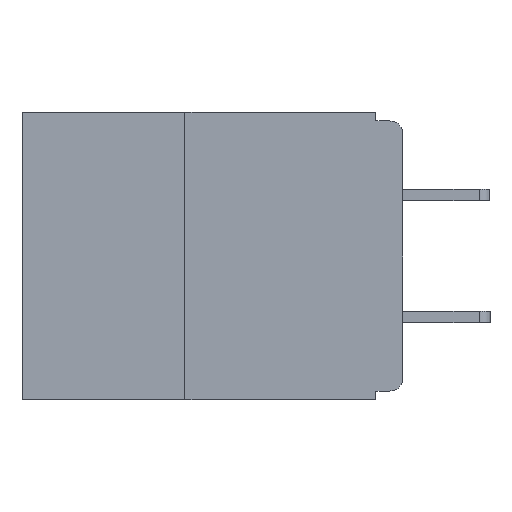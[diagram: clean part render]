
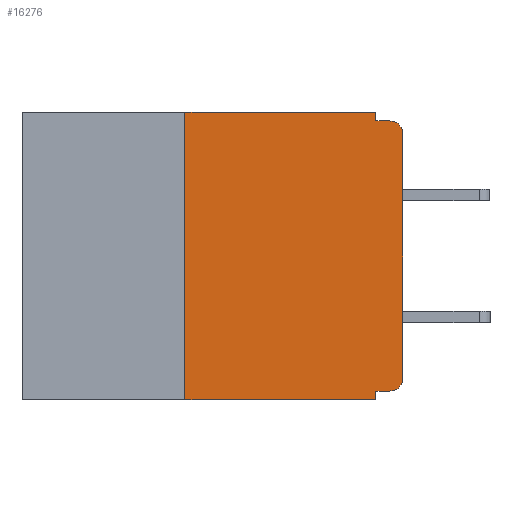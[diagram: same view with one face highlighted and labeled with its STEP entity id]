
A CAD part, left-side view. The second image highlights one B-rep face of the part: STEP entity #16276.
In plain terms, the highlighted planar face has unit normal (-1, 0, 0).
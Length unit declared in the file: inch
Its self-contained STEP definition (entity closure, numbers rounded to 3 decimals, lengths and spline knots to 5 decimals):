
#158 = CARTESIAN_POINT ( 'NONE',  ( 0., 0., -0.32 ) ) ;
#183 = VERTEX_POINT ( 'NONE', #25797 ) ;
#753 = VECTOR ( 'NONE', #14647, 39.37008 ) ;
#823 = DIRECTION ( 'NONE',  ( 0., 0., 1. ) ) ;
#882 = CARTESIAN_POINT ( 'NONE',  ( 0., 0.25, -0.33 ) ) ;
#930 = DIRECTION ( 'NONE',  ( 0., 0., -1. ) ) ;
#1083 = AXIS2_PLACEMENT_3D ( 'NONE', #5230, #19446, #7281 ) ;
#1275 = EDGE_CURVE ( 'NONE', #183, #2156, #4317, .T. ) ;
#1874 = CARTESIAN_POINT ( 'NONE',  ( 0., 0.031, -0.01 ) ) ;
#2099 = ORIENTED_EDGE ( 'NONE', *, *, #3754, .F. ) ;
#2156 = VERTEX_POINT ( 'NONE', #15948 ) ;
#2286 = DIRECTION ( 'NONE',  ( 0., 1., 0. ) ) ;
#2629 = CARTESIAN_POINT ( 'NONE',  ( 0., 0.031, -0.33 ) ) ;
#2714 = CARTESIAN_POINT ( 'NONE',  ( 0., 0.25, 0. ) ) ;
#3185 = LINE ( 'NONE', #158, #13407 ) ;
#3301 = CARTESIAN_POINT ( 'NONE',  ( 0., 0.031, 0. ) ) ;
#3754 = EDGE_CURVE ( 'NONE', #14753, #25849, #5855, .T. ) ;
#4015 = ORIENTED_EDGE ( 'NONE', *, *, #21060, .T. ) ;
#4317 = LINE ( 'NONE', #10270, #753 ) ;
#5230 = CARTESIAN_POINT ( 'NONE',  ( 0., 0.015, -0.305 ) ) ;
#5855 = LINE ( 'NONE', #882, #20406 ) ;
#5869 = CARTESIAN_POINT ( 'NONE',  ( 0., 0.25, -0.33 ) ) ;
#5930 = DIRECTION ( 'NONE',  ( -1., 0., 0. ) ) ;
#6002 = LINE ( 'NONE', #2629, #16252 ) ;
#6218 = VECTOR ( 'NONE', #20703, 39.37008 ) ;
#6501 = CARTESIAN_POINT ( 'NONE',  ( 0., 0.031, 0. ) ) ;
#6821 = VERTEX_POINT ( 'NONE', #1874 ) ;
#7281 = DIRECTION ( 'NONE',  ( 0., 0., -1. ) ) ;
#7584 = EDGE_LOOP ( 'NONE', ( #13887, #15177, #20499, #15820, #17060, #2099, #13587, #18942, #24813, #4015 ) ) ;
#7637 = EDGE_CURVE ( 'NONE', #21924, #6821, #22413, .T. ) ;
#8356 = DIRECTION ( 'NONE',  ( 0., -1., 0. ) ) ;
#9573 = VERTEX_POINT ( 'NONE', #18866 ) ;
#9849 = CARTESIAN_POINT ( 'NONE',  ( 0., 0.015, -0.32 ) ) ;
#10270 = CARTESIAN_POINT ( 'NONE',  ( 0., 0., 0. ) ) ;
#11646 = VECTOR ( 'NONE', #20568, 39.37008 ) ;
#11738 = CARTESIAN_POINT ( 'NONE',  ( 0., 0.437, 0. ) ) ;
#12788 = DIRECTION ( 'NONE',  ( 0., 0., -1. ) ) ;
#13113 = CARTESIAN_POINT ( 'NONE',  ( 0., 0.437, 0. ) ) ;
#13200 = DIRECTION ( 'NONE',  ( 1., 0., 0. ) ) ;
#13407 = VECTOR ( 'NONE', #2286, 39.37008 ) ;
#13587 = ORIENTED_EDGE ( 'NONE', *, *, #16725, .T. ) ;
#13755 = VECTOR ( 'NONE', #8356, 39.37008 ) ;
#13811 = DIRECTION ( 'NONE',  ( 0., -1., 0. ) ) ;
#13869 = VECTOR ( 'NONE', #13811, 39.37008 ) ;
#13887 = ORIENTED_EDGE ( 'NONE', *, *, #1275, .T. ) ;
#14199 = EDGE_CURVE ( 'NONE', #25571, #22318, #3185, .T. ) ;
#14305 = EDGE_CURVE ( 'NONE', #22318, #20951, #6002, .T. ) ;
#14458 = AXIS2_PLACEMENT_3D ( 'NONE', #18157, #5930, #20167 ) ;
#14647 = DIRECTION ( 'NONE',  ( 0., 0., 1. ) ) ;
#14753 = VERTEX_POINT ( 'NONE', #5869 ) ;
#15177 = ORIENTED_EDGE ( 'NONE', *, *, #20674, .T. ) ;
#15820 = ORIENTED_EDGE ( 'NONE', *, *, #7637, .F. ) ;
#15948 = CARTESIAN_POINT ( 'NONE',  ( 0., 0., -0.025 ) ) ;
#16252 = VECTOR ( 'NONE', #12788, 39.37008 ) ;
#16276 = ADVANCED_FACE ( 'NONE', ( #23008 ), #21211, .F. ) ;
#16725 = EDGE_CURVE ( 'NONE', #14753, #20951, #22383, .T. ) ;
#16909 = CARTESIAN_POINT ( 'NONE',  ( 0., 0.031, -0.33 ) ) ;
#17060 = ORIENTED_EDGE ( 'NONE', *, *, #18411, .F. ) ;
#17937 = AXIS2_PLACEMENT_3D ( 'NONE', #13113, #13200, #930 ) ;
#18157 = CARTESIAN_POINT ( 'NONE',  ( 0., 0.015, -0.025 ) ) ;
#18411 = EDGE_CURVE ( 'NONE', #25849, #21924, #19230, .T. ) ;
#18866 = CARTESIAN_POINT ( 'NONE',  ( 0., 0.015, -0.01 ) ) ;
#18942 = ORIENTED_EDGE ( 'NONE', *, *, #14305, .F. ) ;
#19081 = CIRCLE ( 'NONE', #1083, 0.015 ) ;
#19107 = LINE ( 'NONE', #24436, #13755 ) ;
#19230 = LINE ( 'NONE', #11738, #13869 ) ;
#19446 = DIRECTION ( 'NONE',  ( -1., 0., 0. ) ) ;
#20167 = DIRECTION ( 'NONE',  ( 0., 0., -1. ) ) ;
#20406 = VECTOR ( 'NONE', #823, 39.37008 ) ;
#20499 = ORIENTED_EDGE ( 'NONE', *, *, #21326, .F. ) ;
#20568 = DIRECTION ( 'NONE',  ( 0., -1., 0. ) ) ;
#20674 = EDGE_CURVE ( 'NONE', #2156, #9573, #23139, .T. ) ;
#20703 = DIRECTION ( 'NONE',  ( 0., 0., -1. ) ) ;
#20834 = CARTESIAN_POINT ( 'NONE',  ( 0., 0.031, -0.32 ) ) ;
#20951 = VERTEX_POINT ( 'NONE', #16909 ) ;
#21060 = EDGE_CURVE ( 'NONE', #25571, #183, #19081, .T. ) ;
#21211 = PLANE ( 'NONE',  #17937 ) ;
#21326 = EDGE_CURVE ( 'NONE', #6821, #9573, #19107, .T. ) ;
#21924 = VERTEX_POINT ( 'NONE', #3301 ) ;
#22318 = VERTEX_POINT ( 'NONE', #20834 ) ;
#22383 = LINE ( 'NONE', #22574, #11646 ) ;
#22413 = LINE ( 'NONE', #6501, #6218 ) ;
#22574 = CARTESIAN_POINT ( 'NONE',  ( 0., 0.437, -0.33 ) ) ;
#23008 = FACE_OUTER_BOUND ( 'NONE', #7584, .T. ) ;
#23139 = CIRCLE ( 'NONE', #14458, 0.015 ) ;
#24436 = CARTESIAN_POINT ( 'NONE',  ( 0., 0., -0.01 ) ) ;
#24813 = ORIENTED_EDGE ( 'NONE', *, *, #14199, .F. ) ;
#25571 = VERTEX_POINT ( 'NONE', #9849 ) ;
#25797 = CARTESIAN_POINT ( 'NONE',  ( 0., 0., -0.305 ) ) ;
#25849 = VERTEX_POINT ( 'NONE', #2714 ) ;
